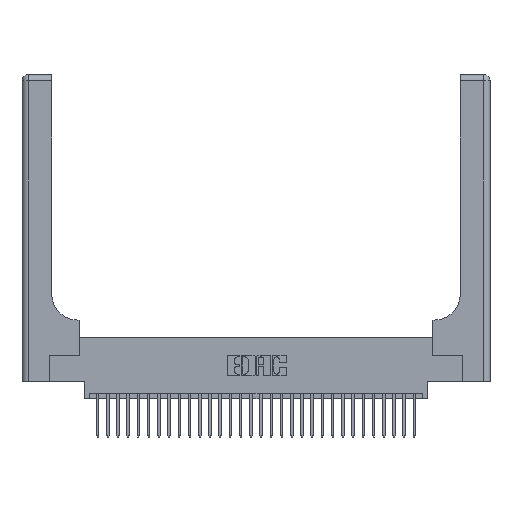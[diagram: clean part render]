
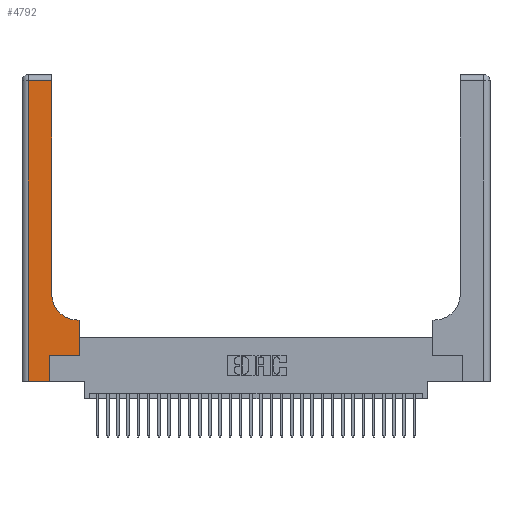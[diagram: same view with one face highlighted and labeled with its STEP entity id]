
A CAD part, top view. The second image highlights one B-rep face of the part: STEP entity #4792.
In plain terms, the highlighted planar face has unit normal (0, 0, 1).
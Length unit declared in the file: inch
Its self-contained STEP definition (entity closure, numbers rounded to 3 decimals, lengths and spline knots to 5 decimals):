
#27 = LINE ( 'NONE', #6910, #25478 ) ;
#1057 = EDGE_CURVE ( 'NONE', #4019, #21857, #13839, .T. ) ;
#2616 = CARTESIAN_POINT ( 'NONE',  ( 0.06, 3., 0.37 ) ) ;
#2633 = ORIENTED_EDGE ( 'NONE', *, *, #13843, .T. ) ;
#2987 = DIRECTION ( 'NONE',  ( -1., 0., 0. ) ) ;
#3060 = LINE ( 'NONE', #2616, #15472 ) ;
#3369 = CARTESIAN_POINT ( 'NONE',  ( 0.2915, 0.6, 0.37 ) ) ;
#3598 = DIRECTION ( 'NONE',  ( -1., 0., 0. ) ) ;
#4019 = VERTEX_POINT ( 'NONE', #27786 ) ;
#4547 = EDGE_CURVE ( 'NONE', #19889, #31137, #27, .T. ) ;
#4792 = ADVANCED_FACE ( 'NONE', ( #25091 ), #29941, .F. ) ;
#4815 = CARTESIAN_POINT ( 'NONE',  ( 0.269, 0., 0.37 ) ) ;
#5039 = AXIS2_PLACEMENT_3D ( 'NONE', #22407, #7618, #24846 ) ;
#5405 = EDGE_CURVE ( 'NONE', #12584, #4019, #3060, .T. ) ;
#5527 = ORIENTED_EDGE ( 'NONE', *, *, #28608, .T. ) ;
#6021 = LINE ( 'NONE', #21972, #19157 ) ;
#6447 = AXIS2_PLACEMENT_3D ( 'NONE', #15342, #17830, #2987 ) ;
#6530 = ORIENTED_EDGE ( 'NONE', *, *, #7405, .T. ) ;
#6541 = LINE ( 'NONE', #4815, #25406 ) ;
#6816 = ORIENTED_EDGE ( 'NONE', *, *, #27325, .T. ) ;
#6910 = CARTESIAN_POINT ( 'NONE',  ( 0.5585, 0.25, 0.37 ) ) ;
#7227 = VECTOR ( 'NONE', #14206, 39.37008 ) ;
#7273 = DIRECTION ( 'NONE',  ( 0., 1., 0. ) ) ;
#7405 = EDGE_CURVE ( 'NONE', #21040, #12584, #6021, .T. ) ;
#7597 = DIRECTION ( 'NONE',  ( 0., -1., 0. ) ) ;
#7618 = DIRECTION ( 'NONE',  ( 0., 0., -1. ) ) ;
#7888 = EDGE_LOOP ( 'NONE', ( #6816, #6530, #17279, #30650, #2633, #13598, #22468, #5527, #24956 ) ) ;
#9403 = DIRECTION ( 'NONE',  ( 0., 1., 0. ) ) ;
#9684 = DIRECTION ( 'NONE',  ( -1., 0., 0. ) ) ;
#10167 = LINE ( 'NONE', #3369, #16000 ) ;
#10238 = CARTESIAN_POINT ( 'NONE',  ( 0.2915, 0.85, 0.37 ) ) ;
#10347 = VERTEX_POINT ( 'NONE', #10238 ) ;
#11054 = CARTESIAN_POINT ( 'NONE',  ( 0.2915, 2.94, 0.37 ) ) ;
#11451 = CARTESIAN_POINT ( 'NONE',  ( 0.5585, 0.25, 0.37 ) ) ;
#12584 = VERTEX_POINT ( 'NONE', #25905 ) ;
#12678 = CARTESIAN_POINT ( 'NONE',  ( 0.5585, 0.6, 0.37 ) ) ;
#13070 = DIRECTION ( 'NONE',  ( 1., 0., 0. ) ) ;
#13174 = LINE ( 'NONE', #17924, #18943 ) ;
#13378 = EDGE_CURVE ( 'NONE', #31667, #19889, #13174, .T. ) ;
#13598 = ORIENTED_EDGE ( 'NONE', *, *, #13378, .T. ) ;
#13839 = LINE ( 'NONE', #14145, #7227 ) ;
#13843 = EDGE_CURVE ( 'NONE', #21857, #31667, #6541, .T. ) ;
#14145 = CARTESIAN_POINT ( 'NONE',  ( 0., 0., 0.37 ) ) ;
#14206 = DIRECTION ( 'NONE',  ( 1., 0., 0. ) ) ;
#15342 = CARTESIAN_POINT ( 'NONE',  ( 0., 3., 0.37 ) ) ;
#15472 = VECTOR ( 'NONE', #7597, 39.37008 ) ;
#16000 = VECTOR ( 'NONE', #3598, 39.37008 ) ;
#17279 = ORIENTED_EDGE ( 'NONE', *, *, #5405, .T. ) ;
#17625 = CARTESIAN_POINT ( 'NONE',  ( 0.5415, 0.6, 0.37 ) ) ;
#17830 = DIRECTION ( 'NONE',  ( 0., 0., -1. ) ) ;
#17924 = CARTESIAN_POINT ( 'NONE',  ( 0.269, 0.25, 0.37 ) ) ;
#18280 = EDGE_CURVE ( 'NONE', #24001, #10347, #20223, .T. ) ;
#18774 = VECTOR ( 'NONE', #30179, 39.37008 ) ;
#18811 = CARTESIAN_POINT ( 'NONE',  ( 0.269, 0., 0.37 ) ) ;
#18943 = VECTOR ( 'NONE', #13070, 39.37008 ) ;
#19157 = VECTOR ( 'NONE', #9684, 39.37008 ) ;
#19758 = CARTESIAN_POINT ( 'NONE',  ( 0.269, 0.25, 0.37 ) ) ;
#19889 = VERTEX_POINT ( 'NONE', #11451 ) ;
#20223 = CIRCLE ( 'NONE', #5039, 0.25 ) ;
#21040 = VERTEX_POINT ( 'NONE', #11054 ) ;
#21857 = VERTEX_POINT ( 'NONE', #18811 ) ;
#21972 = CARTESIAN_POINT ( 'NONE',  ( 0., 2.94, 0.37 ) ) ;
#22407 = CARTESIAN_POINT ( 'NONE',  ( 0.5415, 0.85, 0.37 ) ) ;
#22468 = ORIENTED_EDGE ( 'NONE', *, *, #4547, .T. ) ;
#22862 = CARTESIAN_POINT ( 'NONE',  ( 0.2915, 3., 0.37 ) ) ;
#24001 = VERTEX_POINT ( 'NONE', #17625 ) ;
#24846 = DIRECTION ( 'NONE',  ( 1., 0., 0. ) ) ;
#24956 = ORIENTED_EDGE ( 'NONE', *, *, #18280, .T. ) ;
#25091 = FACE_OUTER_BOUND ( 'NONE', #7888, .T. ) ;
#25406 = VECTOR ( 'NONE', #7273, 39.37008 ) ;
#25478 = VECTOR ( 'NONE', #9403, 39.37008 ) ;
#25905 = CARTESIAN_POINT ( 'NONE',  ( 0.06, 2.94, 0.37 ) ) ;
#26757 = LINE ( 'NONE', #22862, #18774 ) ;
#27325 = EDGE_CURVE ( 'NONE', #10347, #21040, #26757, .T. ) ;
#27786 = CARTESIAN_POINT ( 'NONE',  ( 0.06, 0., 0.37 ) ) ;
#28608 = EDGE_CURVE ( 'NONE', #31137, #24001, #10167, .T. ) ;
#29941 = PLANE ( 'NONE',  #6447 ) ;
#30179 = DIRECTION ( 'NONE',  ( 0., 1., 0. ) ) ;
#30650 = ORIENTED_EDGE ( 'NONE', *, *, #1057, .T. ) ;
#31137 = VERTEX_POINT ( 'NONE', #12678 ) ;
#31667 = VERTEX_POINT ( 'NONE', #19758 ) ;
